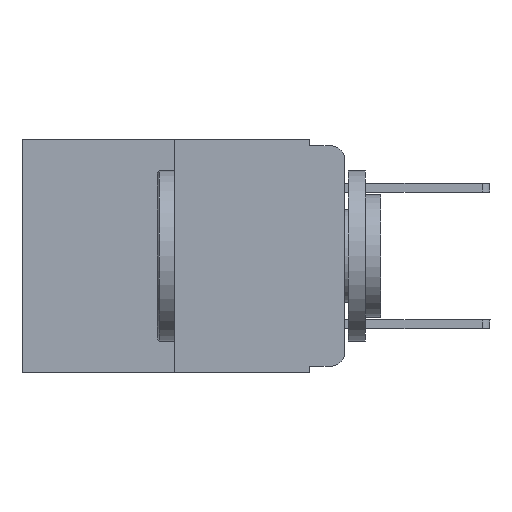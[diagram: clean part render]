
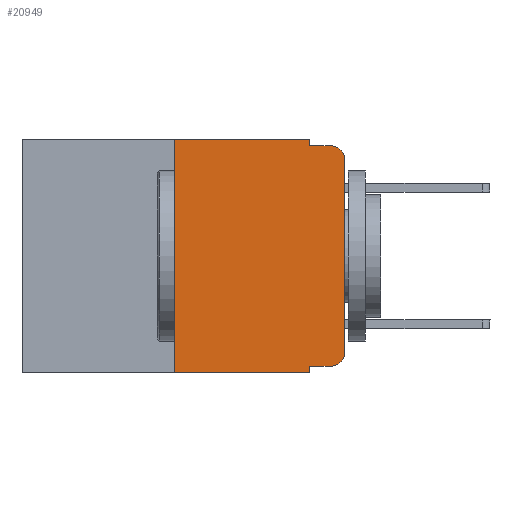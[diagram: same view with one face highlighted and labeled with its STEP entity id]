
A CAD part, left-side view. The second image highlights one B-rep face of the part: STEP entity #20949.
In plain terms, the highlighted planar face has unit normal (-1, 0, 0).
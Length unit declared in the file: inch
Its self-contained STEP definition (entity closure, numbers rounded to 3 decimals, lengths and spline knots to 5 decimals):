
#44 = EDGE_CURVE ( 'NONE', #5236, #9232, #8507, .T. ) ;
#370 = EDGE_CURVE ( 'NONE', #10852, #12229, #1503, .T. ) ;
#524 = LINE ( 'NONE', #8909, #17887 ) ;
#743 = EDGE_CURVE ( 'NONE', #11497, #10852, #5112, .T. ) ;
#1047 = CIRCLE ( 'NONE', #13643, 0.02 ) ;
#1053 = EDGE_CURVE ( 'NONE', #9232, #11497, #1047, .T. ) ;
#1503 = CIRCLE ( 'NONE', #7632, 0.02 ) ;
#1888 = DIRECTION ( 'NONE',  ( 0., 0., -1. ) ) ;
#2061 = CARTESIAN_POINT ( 'NONE',  ( 0., 0., -0.313 ) ) ;
#2183 = EDGE_CURVE ( 'NONE', #17042, #19624, #19921, .T. ) ;
#2358 = CARTESIAN_POINT ( 'NONE',  ( 0., 0.25, 0. ) ) ;
#2401 = ORIENTED_EDGE ( 'NONE', *, *, #1053, .T. ) ;
#2492 = PLANE ( 'NONE',  #17893 ) ;
#2683 = DIRECTION ( 'NONE',  ( -1., 0., 0. ) ) ;
#2719 = VERTEX_POINT ( 'NONE', #9481 ) ;
#3168 = CARTESIAN_POINT ( 'NONE',  ( 0., 0., -0.03 ) ) ;
#3709 = VERTEX_POINT ( 'NONE', #13881 ) ;
#4379 = ORIENTED_EDGE ( 'NONE', *, *, #19819, .F. ) ;
#4402 = EDGE_CURVE ( 'NONE', #19624, #11697, #6357, .T. ) ;
#5015 = VECTOR ( 'NONE', #5134, 39.37008 ) ;
#5112 = LINE ( 'NONE', #8372, #12399 ) ;
#5134 = DIRECTION ( 'NONE',  ( 0., -1., 0. ) ) ;
#5236 = VERTEX_POINT ( 'NONE', #5883 ) ;
#5240 = DIRECTION ( 'NONE',  ( 0., 0., 1. ) ) ;
#5289 = CARTESIAN_POINT ( 'NONE',  ( 0., 0.02, -0.313 ) ) ;
#5883 = CARTESIAN_POINT ( 'NONE',  ( 0., 0.051, -0.333 ) ) ;
#6357 = LINE ( 'NONE', #14667, #21274 ) ;
#7632 = AXIS2_PLACEMENT_3D ( 'NONE', #11575, #2683, #9531 ) ;
#7687 = DIRECTION ( 'NONE',  ( 0., -1., 0. ) ) ;
#7773 = ORIENTED_EDGE ( 'NONE', *, *, #370, .T. ) ;
#8372 = CARTESIAN_POINT ( 'NONE',  ( 0., 0., 0. ) ) ;
#8507 = LINE ( 'NONE', #11889, #5015 ) ;
#8849 = VECTOR ( 'NONE', #13301, 39.37008 ) ;
#8890 = EDGE_CURVE ( 'NONE', #17042, #2719, #18180, .T. ) ;
#8909 = CARTESIAN_POINT ( 'NONE',  ( 0., 0.051, 0. ) ) ;
#9232 = VERTEX_POINT ( 'NONE', #12049 ) ;
#9400 = CARTESIAN_POINT ( 'NONE',  ( 0., 0.02, -0.01 ) ) ;
#9481 = CARTESIAN_POINT ( 'NONE',  ( 0., 0.051, -0.343 ) ) ;
#9531 = DIRECTION ( 'NONE',  ( 0., 0., -1. ) ) ;
#9647 = CARTESIAN_POINT ( 'NONE',  ( 0., 0.25, 0. ) ) ;
#9891 = LINE ( 'NONE', #16760, #10267 ) ;
#10267 = VECTOR ( 'NONE', #16309, 39.37008 ) ;
#10368 = ORIENTED_EDGE ( 'NONE', *, *, #44, .T. ) ;
#10477 = DIRECTION ( 'NONE',  ( 0., 0., -1. ) ) ;
#10702 = ORIENTED_EDGE ( 'NONE', *, *, #743, .T. ) ;
#10852 = VERTEX_POINT ( 'NONE', #3168 ) ;
#10857 = EDGE_CURVE ( 'NONE', #3709, #12229, #16877, .T. ) ;
#11497 = VERTEX_POINT ( 'NONE', #2061 ) ;
#11575 = CARTESIAN_POINT ( 'NONE',  ( 0., 0.02, -0.03 ) ) ;
#11591 = ORIENTED_EDGE ( 'NONE', *, *, #10857, .F. ) ;
#11651 = CARTESIAN_POINT ( 'NONE',  ( 0., 0.051, 0. ) ) ;
#11697 = VERTEX_POINT ( 'NONE', #11651 ) ;
#11848 = EDGE_CURVE ( 'NONE', #11697, #3709, #524, .T. ) ;
#11889 = CARTESIAN_POINT ( 'NONE',  ( 0., 0.051, -0.333 ) ) ;
#12049 = CARTESIAN_POINT ( 'NONE',  ( 0., 0.02, -0.333 ) ) ;
#12229 = VERTEX_POINT ( 'NONE', #9400 ) ;
#12399 = VECTOR ( 'NONE', #15331, 39.37008 ) ;
#12977 = DIRECTION ( 'NONE',  ( 1., 0., 0. ) ) ;
#13058 = EDGE_LOOP ( 'NONE', ( #10702, #7773, #11591, #16532, #21590, #17790, #16539, #4379, #10368, #2401 ) ) ;
#13217 = DIRECTION ( 'NONE',  ( 0., -1., 0. ) ) ;
#13301 = DIRECTION ( 'NONE',  ( 0., -1., 0. ) ) ;
#13643 = AXIS2_PLACEMENT_3D ( 'NONE', #5289, #17561, #1888 ) ;
#13881 = CARTESIAN_POINT ( 'NONE',  ( 0., 0.051, -0.01 ) ) ;
#14667 = CARTESIAN_POINT ( 'NONE',  ( 0., 0.473, 0. ) ) ;
#14687 = VECTOR ( 'NONE', #5240, 39.37008 ) ;
#14780 = CARTESIAN_POINT ( 'NONE',  ( 0., 0.473, -0.343 ) ) ;
#15194 = CARTESIAN_POINT ( 'NONE',  ( 0., 0.051, -0.01 ) ) ;
#15331 = DIRECTION ( 'NONE',  ( 0., 0., 1. ) ) ;
#15859 = CARTESIAN_POINT ( 'NONE',  ( 0., 0.473, 0. ) ) ;
#16309 = DIRECTION ( 'NONE',  ( 0., 0., -1. ) ) ;
#16532 = ORIENTED_EDGE ( 'NONE', *, *, #11848, .F. ) ;
#16539 = ORIENTED_EDGE ( 'NONE', *, *, #8890, .T. ) ;
#16760 = CARTESIAN_POINT ( 'NONE',  ( 0., 0.051, 0. ) ) ;
#16877 = LINE ( 'NONE', #15194, #8849 ) ;
#17042 = VERTEX_POINT ( 'NONE', #17573 ) ;
#17561 = DIRECTION ( 'NONE',  ( -1., 0., 0. ) ) ;
#17573 = CARTESIAN_POINT ( 'NONE',  ( 0., 0.25, -0.343 ) ) ;
#17578 = DIRECTION ( 'NONE',  ( 0., 0., -1. ) ) ;
#17690 = FACE_OUTER_BOUND ( 'NONE', #13058, .T. ) ;
#17790 = ORIENTED_EDGE ( 'NONE', *, *, #2183, .F. ) ;
#17887 = VECTOR ( 'NONE', #10477, 39.37008 ) ;
#17893 = AXIS2_PLACEMENT_3D ( 'NONE', #15859, #12977, #17578 ) ;
#18180 = LINE ( 'NONE', #14780, #21747 ) ;
#19624 = VERTEX_POINT ( 'NONE', #2358 ) ;
#19819 = EDGE_CURVE ( 'NONE', #5236, #2719, #9891, .T. ) ;
#19921 = LINE ( 'NONE', #9647, #14687 ) ;
#20949 = ADVANCED_FACE ( 'NONE', ( #17690 ), #2492, .F. ) ;
#21274 = VECTOR ( 'NONE', #13217, 39.37008 ) ;
#21590 = ORIENTED_EDGE ( 'NONE', *, *, #4402, .F. ) ;
#21747 = VECTOR ( 'NONE', #7687, 39.37008 ) ;
